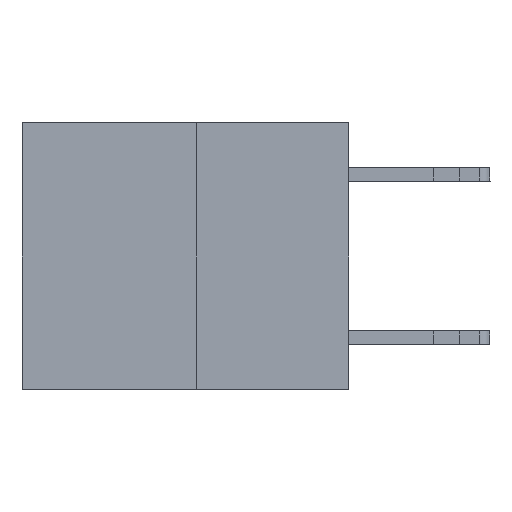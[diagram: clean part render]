
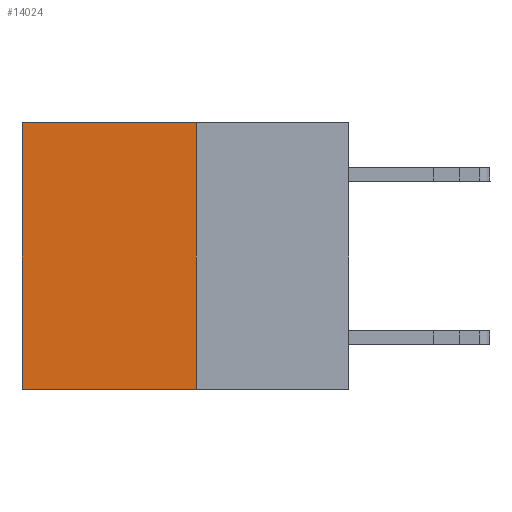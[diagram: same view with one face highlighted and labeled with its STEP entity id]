
A CAD part, left-side view. The second image highlights one B-rep face of the part: STEP entity #14024.
In plain terms, the highlighted planar face has unit normal (-1, 0, 0).
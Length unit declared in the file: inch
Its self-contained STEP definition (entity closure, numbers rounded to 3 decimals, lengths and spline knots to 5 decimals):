
#169 = EDGE_LOOP ( 'NONE', ( #18374, #226, #16086, #4618 ) ) ;
#226 = ORIENTED_EDGE ( 'NONE', *, *, #13189, .F. ) ;
#579 = LINE ( 'NONE', #3946, #2150 ) ;
#793 = EDGE_CURVE ( 'NONE', #18915, #1775, #17321, .T. ) ;
#1394 = CARTESIAN_POINT ( 'NONE',  ( 0.3165, 0.28, -0.49 ) ) ;
#1775 = VERTEX_POINT ( 'NONE', #17808 ) ;
#2150 = VECTOR ( 'NONE', #5433, 39.37008 ) ;
#3946 = CARTESIAN_POINT ( 'NONE',  ( 0.3165, 0.28, -0.49 ) ) ;
#4098 = CARTESIAN_POINT ( 'NONE',  ( 0.3165, 0.28, -0.49 ) ) ;
#4618 = ORIENTED_EDGE ( 'NONE', *, *, #7955, .T. ) ;
#4706 = VECTOR ( 'NONE', #7957, 39.37008 ) ;
#5433 = DIRECTION ( 'NONE',  ( 0., 1., 0. ) ) ;
#5752 = VERTEX_POINT ( 'NONE', #18545 ) ;
#6766 = EDGE_CURVE ( 'NONE', #7958, #5752, #9319, .T. ) ;
#7413 = DIRECTION ( 'NONE',  ( 0., 0., -1. ) ) ;
#7674 = CARTESIAN_POINT ( 'NONE',  ( 0.3165, 0.6, 0. ) ) ;
#7781 = VECTOR ( 'NONE', #10539, 39.37008 ) ;
#7955 = EDGE_CURVE ( 'NONE', #18915, #7958, #16171, .T. ) ;
#7957 = DIRECTION ( 'NONE',  ( 0., 0., -1. ) ) ;
#7958 = VERTEX_POINT ( 'NONE', #7674 ) ;
#8917 = DIRECTION ( 'NONE',  ( 1., 0., 0. ) ) ;
#9103 = CARTESIAN_POINT ( 'NONE',  ( 0.3165, 0.28, 0. ) ) ;
#9319 = LINE ( 'NONE', #10327, #7781 ) ;
#10327 = CARTESIAN_POINT ( 'NONE',  ( 0.3165, 0.6, -0.49 ) ) ;
#10539 = DIRECTION ( 'NONE',  ( 0., 0., -1. ) ) ;
#11160 = AXIS2_PLACEMENT_3D ( 'NONE', #4098, #8917, #7413 ) ;
#13104 = VECTOR ( 'NONE', #15852, 39.37008 ) ;
#13189 = EDGE_CURVE ( 'NONE', #1775, #5752, #579, .T. ) ;
#14024 = ADVANCED_FACE ( 'NONE', ( #20398 ), #16953, .F. ) ;
#15852 = DIRECTION ( 'NONE',  ( 0., 1., 0. ) ) ;
#16086 = ORIENTED_EDGE ( 'NONE', *, *, #793, .F. ) ;
#16171 = LINE ( 'NONE', #9103, #13104 ) ;
#16953 = PLANE ( 'NONE',  #11160 ) ;
#17321 = LINE ( 'NONE', #1394, #4706 ) ;
#17808 = CARTESIAN_POINT ( 'NONE',  ( 0.3165, 0.28, -0.49 ) ) ;
#18374 = ORIENTED_EDGE ( 'NONE', *, *, #6766, .T. ) ;
#18383 = CARTESIAN_POINT ( 'NONE',  ( 0.3165, 0.28, 0. ) ) ;
#18545 = CARTESIAN_POINT ( 'NONE',  ( 0.3165, 0.6, -0.49 ) ) ;
#18915 = VERTEX_POINT ( 'NONE', #18383 ) ;
#20398 = FACE_OUTER_BOUND ( 'NONE', #169, .T. ) ;
